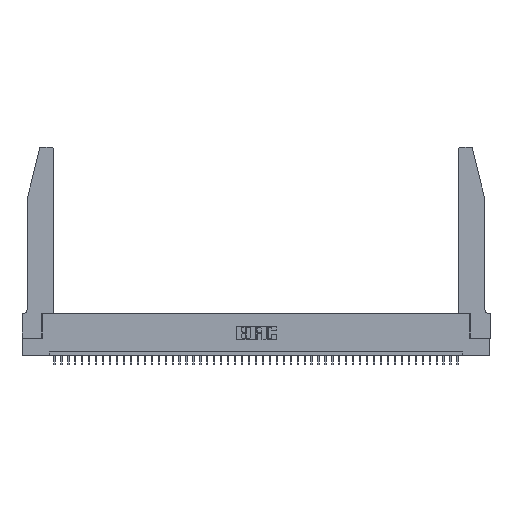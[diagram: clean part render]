
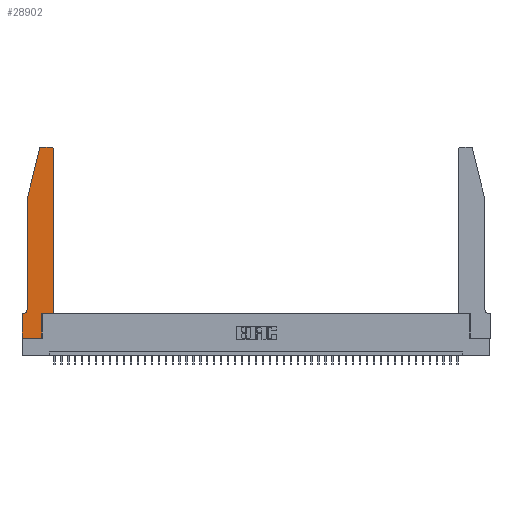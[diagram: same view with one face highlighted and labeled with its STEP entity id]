
A CAD part, top view. The second image highlights one B-rep face of the part: STEP entity #28902.
In plain terms, the highlighted planar face has unit normal (0, 0, 1).
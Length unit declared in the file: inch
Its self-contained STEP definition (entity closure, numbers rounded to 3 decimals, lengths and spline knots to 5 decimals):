
#250 = DIRECTION ( 'NONE',  ( 1., 0., 0. ) ) ;
#694 = LINE ( 'NONE', #33915, #1415 ) ;
#827 = CARTESIAN_POINT ( 'NONE',  ( 0.2865, 0., 0.37 ) ) ;
#1296 = CARTESIAN_POINT ( 'NONE',  ( 0.4505, 0.35, 0.37 ) ) ;
#1415 = VECTOR ( 'NONE', #4469, 39.37008 ) ;
#2890 = DIRECTION ( 'NONE',  ( -1., 0., 0. ) ) ;
#3794 = VECTOR ( 'NONE', #26174, 39.37008 ) ;
#4469 = DIRECTION ( 'NONE',  ( -1., 0., 0. ) ) ;
#4822 = CARTESIAN_POINT ( 'NONE',  ( 0., 0., 0.37 ) ) ;
#5049 = CARTESIAN_POINT ( 'NONE',  ( 0.4505, 0.35, 0.37 ) ) ;
#5135 = EDGE_CURVE ( 'NONE', #32370, #45017, #16087, .T. ) ;
#5241 = CARTESIAN_POINT ( 'NONE',  ( 0.284, 2.75, 0.37 ) ) ;
#5579 = VERTEX_POINT ( 'NONE', #22890 ) ;
#5661 = CARTESIAN_POINT ( 'NONE',  ( 0., 0., 0.37 ) ) ;
#5830 = CARTESIAN_POINT ( 'NONE',  ( 0., 0., 0.37 ) ) ;
#5991 = AXIS2_PLACEMENT_3D ( 'NONE', #21640, #10482, #36102 ) ;
#7578 = VERTEX_POINT ( 'NONE', #827 ) ;
#9542 = ORIENTED_EDGE ( 'NONE', *, *, #28328, .T. ) ;
#9953 = FACE_OUTER_BOUND ( 'NONE', #35152, .T. ) ;
#10482 = DIRECTION ( 'NONE',  ( 0., 0., -1. ) ) ;
#11168 = VECTOR ( 'NONE', #25647, 39.37008 ) ;
#11375 = EDGE_CURVE ( 'NONE', #22069, #38670, #18072, .T. ) ;
#12090 = EDGE_CURVE ( 'NONE', #21122, #15560, #694, .T. ) ;
#12417 = DIRECTION ( 'NONE',  ( 1., 0., 0. ) ) ;
#12955 = DIRECTION ( 'NONE',  ( 0., -1., 0. ) ) ;
#13203 = EDGE_CURVE ( 'NONE', #38670, #21122, #46095, .T. ) ;
#13768 = VECTOR ( 'NONE', #12955, 39.37008 ) ;
#13792 = LINE ( 'NONE', #39435, #26309 ) ;
#13893 = EDGE_CURVE ( 'NONE', #29248, #7578, #30544, .T. ) ;
#14220 = VECTOR ( 'NONE', #32094, 39.37008 ) ;
#15182 = VERTEX_POINT ( 'NONE', #41153 ) ;
#15244 = ORIENTED_EDGE ( 'NONE', *, *, #31706, .T. ) ;
#15560 = VERTEX_POINT ( 'NONE', #5241 ) ;
#15848 = CARTESIAN_POINT ( 'NONE',  ( 0.0755, 2., 0.37 ) ) ;
#16074 = DIRECTION ( 'NONE',  ( 1., 0., 0. ) ) ;
#16087 = LINE ( 'NONE', #15848, #13768 ) ;
#16616 = CIRCLE ( 'NONE', #5991, 0.07 ) ;
#17032 = VERTEX_POINT ( 'NONE', #44396 ) ;
#17339 = CARTESIAN_POINT ( 'NONE',  ( 0.4205, 2.72, 0.37 ) ) ;
#18072 = LINE ( 'NONE', #39446, #14220 ) ;
#19268 = LINE ( 'NONE', #43718, #11168 ) ;
#19651 = VECTOR ( 'NONE', #12417, 39.37008 ) ;
#19735 = PLANE ( 'NONE',  #29545 ) ;
#21030 = CARTESIAN_POINT ( 'NONE',  ( 0.25487, 2.72718, 0.37 ) ) ;
#21122 = VERTEX_POINT ( 'NONE', #44149 ) ;
#21352 = DIRECTION ( 'NONE',  ( 1., 0., 0. ) ) ;
#21640 = CARTESIAN_POINT ( 'NONE',  ( 0.0055, 0.42, 0.37 ) ) ;
#21682 = DIRECTION ( 'NONE',  ( 0., 1., 0. ) ) ;
#21961 = VECTOR ( 'NONE', #16074, 39.37008 ) ;
#22069 = VERTEX_POINT ( 'NONE', #5049 ) ;
#22622 = CARTESIAN_POINT ( 'NONE',  ( 0.2865, 0.35, 0.37 ) ) ;
#22661 = CARTESIAN_POINT ( 'NONE',  ( 0.4505, 2.72, 0.37 ) ) ;
#22890 = CARTESIAN_POINT ( 'NONE',  ( 0., 0.35, 0.37 ) ) ;
#23819 = EDGE_CURVE ( 'NONE', #41411, #32370, #19268, .T. ) ;
#24247 = ORIENTED_EDGE ( 'NONE', *, *, #26861, .T. ) ;
#25089 = ORIENTED_EDGE ( 'NONE', *, *, #46003, .T. ) ;
#25647 = DIRECTION ( 'NONE',  ( -0.239, -0.971, 0. ) ) ;
#25927 = LINE ( 'NONE', #4822, #3794 ) ;
#25946 = LINE ( 'NONE', #1296, #19651 ) ;
#26174 = DIRECTION ( 'NONE',  ( 0., -1., 0. ) ) ;
#26309 = VECTOR ( 'NONE', #2890, 39.37008 ) ;
#26861 = EDGE_CURVE ( 'NONE', #17032, #22069, #25946, .T. ) ;
#27081 = AXIS2_PLACEMENT_3D ( 'NONE', #17339, #39861, #250 ) ;
#27388 = CARTESIAN_POINT ( 'NONE',  ( 0.284, 2.72, 0.37 ) ) ;
#28066 = DIRECTION ( 'NONE',  ( 0., 0., 1. ) ) ;
#28328 = EDGE_CURVE ( 'NONE', #15560, #41411, #37102, .T. ) ;
#28444 = ORIENTED_EDGE ( 'NONE', *, *, #11375, .T. ) ;
#28902 = ADVANCED_FACE ( 'NONE', ( #9953 ), #19735, .T. ) ;
#29248 = VERTEX_POINT ( 'NONE', #5661 ) ;
#29417 = ORIENTED_EDGE ( 'NONE', *, *, #23819, .T. ) ;
#29545 = AXIS2_PLACEMENT_3D ( 'NONE', #35605, #31807, #21352 ) ;
#30544 = LINE ( 'NONE', #5830, #21961 ) ;
#31204 = VECTOR ( 'NONE', #21682, 39.37008 ) ;
#31619 = DIRECTION ( 'NONE',  ( 1., 0., 0. ) ) ;
#31706 = EDGE_CURVE ( 'NONE', #7578, #17032, #36843, .T. ) ;
#31807 = DIRECTION ( 'NONE',  ( 0., 0., 1. ) ) ;
#32094 = DIRECTION ( 'NONE',  ( 0., 1., 0. ) ) ;
#32370 = VERTEX_POINT ( 'NONE', #38460 ) ;
#32528 = ORIENTED_EDGE ( 'NONE', *, *, #41828, .T. ) ;
#33055 = ORIENTED_EDGE ( 'NONE', *, *, #5135, .T. ) ;
#33915 = CARTESIAN_POINT ( 'NONE',  ( 0.2605, 2.75, 0.37 ) ) ;
#35152 = EDGE_LOOP ( 'NONE', ( #36520, #9542, #29417, #33055, #36717, #32528, #25089, #37441, #15244, #24247, #28444, #35540 ) ) ;
#35540 = ORIENTED_EDGE ( 'NONE', *, *, #13203, .T. ) ;
#35605 = CARTESIAN_POINT ( 'NONE',  ( 0., 0.35, 0.37 ) ) ;
#36102 = DIRECTION ( 'NONE',  ( -1., 0., 0. ) ) ;
#36520 = ORIENTED_EDGE ( 'NONE', *, *, #12090, .T. ) ;
#36717 = ORIENTED_EDGE ( 'NONE', *, *, #44886, .T. ) ;
#36843 = LINE ( 'NONE', #22622, #31204 ) ;
#37102 = CIRCLE ( 'NONE', #43199, 0.03 ) ;
#37441 = ORIENTED_EDGE ( 'NONE', *, *, #13893, .T. ) ;
#38460 = CARTESIAN_POINT ( 'NONE',  ( 0.0755, 2., 0.37 ) ) ;
#38670 = VERTEX_POINT ( 'NONE', #22661 ) ;
#39435 = CARTESIAN_POINT ( 'NONE',  ( 0.0755, 0.35, 0.37 ) ) ;
#39446 = CARTESIAN_POINT ( 'NONE',  ( 0.4505, 0.35, 0.37 ) ) ;
#39861 = DIRECTION ( 'NONE',  ( 0., 0., 1. ) ) ;
#41153 = CARTESIAN_POINT ( 'NONE',  ( 0.0055, 0.35, 0.37 ) ) ;
#41411 = VERTEX_POINT ( 'NONE', #21030 ) ;
#41828 = EDGE_CURVE ( 'NONE', #15182, #5579, #13792, .T. ) ;
#43199 = AXIS2_PLACEMENT_3D ( 'NONE', #27388, #28066, #31619 ) ;
#43718 = CARTESIAN_POINT ( 'NONE',  ( 0.0755, 2., 0.37 ) ) ;
#44149 = CARTESIAN_POINT ( 'NONE',  ( 0.4205, 2.75, 0.37 ) ) ;
#44396 = CARTESIAN_POINT ( 'NONE',  ( 0.2865, 0.35, 0.37 ) ) ;
#44444 = CARTESIAN_POINT ( 'NONE',  ( 0.0755, 0.42, 0.37 ) ) ;
#44886 = EDGE_CURVE ( 'NONE', #45017, #15182, #16616, .T. ) ;
#45017 = VERTEX_POINT ( 'NONE', #44444 ) ;
#46003 = EDGE_CURVE ( 'NONE', #5579, #29248, #25927, .T. ) ;
#46095 = CIRCLE ( 'NONE', #27081, 0.03 ) ;
